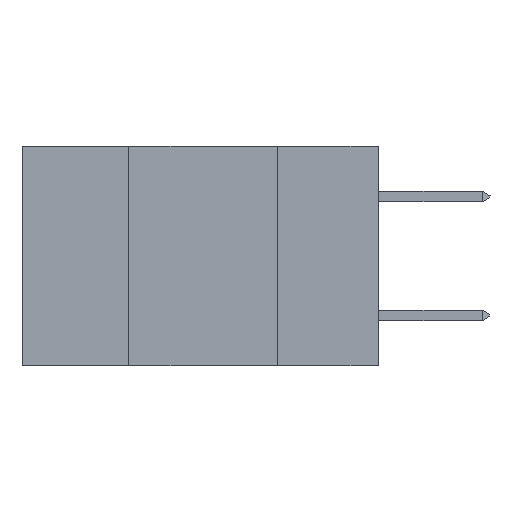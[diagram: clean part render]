
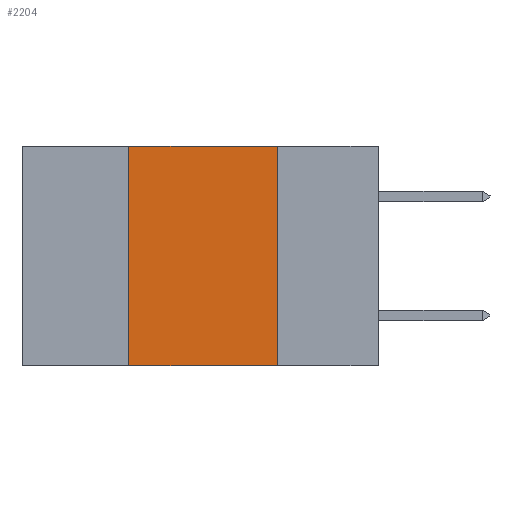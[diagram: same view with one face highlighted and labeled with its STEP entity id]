
A CAD part, left-side view. The second image highlights one B-rep face of the part: STEP entity #2204.
In plain terms, the highlighted planar face has unit normal (-1, 0, 0).
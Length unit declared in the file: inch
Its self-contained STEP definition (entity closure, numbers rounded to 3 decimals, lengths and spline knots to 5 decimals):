
#154 = ORIENTED_EDGE ( 'NONE', *, *, #9195, .F. ) ;
#379 = DIRECTION ( 'NONE',  ( 0., 0., 1. ) ) ;
#557 = EDGE_CURVE ( 'NONE', #3287, #9717, #8449, .T. ) ;
#773 = VECTOR ( 'NONE', #4101, 39.37008 ) ;
#999 = LINE ( 'NONE', #1804, #9194 ) ;
#1150 = DIRECTION ( 'NONE',  ( 0., 0., -1. ) ) ;
#1745 = DIRECTION ( 'NONE',  ( 0., -1., 0. ) ) ;
#1804 = CARTESIAN_POINT ( 'NONE',  ( 0., 0.6, -0.37 ) ) ;
#1882 = EDGE_LOOP ( 'NONE', ( #5538, #154, #5815, #4327 ) ) ;
#2204 = ADVANCED_FACE ( 'NONE', ( #4510 ), #5127, .F. ) ;
#2981 = VECTOR ( 'NONE', #5405, 39.37008 ) ;
#3287 = VERTEX_POINT ( 'NONE', #4253 ) ;
#4101 = DIRECTION ( 'NONE',  ( 0., -1., 0. ) ) ;
#4253 = CARTESIAN_POINT ( 'NONE',  ( 0., 0.42, -0.37 ) ) ;
#4327 = ORIENTED_EDGE ( 'NONE', *, *, #5433, .T. ) ;
#4399 = CARTESIAN_POINT ( 'NONE',  ( 0., 0.6, 0. ) ) ;
#4510 = FACE_OUTER_BOUND ( 'NONE', #1882, .T. ) ;
#4608 = VECTOR ( 'NONE', #379, 39.37008 ) ;
#4949 = VERTEX_POINT ( 'NONE', #4991 ) ;
#4969 = LINE ( 'NONE', #8846, #773 ) ;
#4991 = CARTESIAN_POINT ( 'NONE',  ( 0., 0.17, -0.37 ) ) ;
#5051 = AXIS2_PLACEMENT_3D ( 'NONE', #4399, #8329, #1150 ) ;
#5127 = PLANE ( 'NONE',  #5051 ) ;
#5405 = DIRECTION ( 'NONE',  ( 0., 0., -1. ) ) ;
#5433 = EDGE_CURVE ( 'NONE', #3287, #4949, #999, .T. ) ;
#5538 = ORIENTED_EDGE ( 'NONE', *, *, #9918, .F. ) ;
#5815 = ORIENTED_EDGE ( 'NONE', *, *, #557, .F. ) ;
#6698 = VERTEX_POINT ( 'NONE', #9164 ) ;
#8329 = DIRECTION ( 'NONE',  ( 1., 0., 0. ) ) ;
#8449 = LINE ( 'NONE', #10059, #4608 ) ;
#8752 = LINE ( 'NONE', #10229, #2981 ) ;
#8846 = CARTESIAN_POINT ( 'NONE',  ( 0., 0.6, 0. ) ) ;
#9127 = CARTESIAN_POINT ( 'NONE',  ( 0., 0.42, 0. ) ) ;
#9164 = CARTESIAN_POINT ( 'NONE',  ( 0., 0.17, 0. ) ) ;
#9194 = VECTOR ( 'NONE', #1745, 39.37008 ) ;
#9195 = EDGE_CURVE ( 'NONE', #9717, #6698, #4969, .T. ) ;
#9717 = VERTEX_POINT ( 'NONE', #9127 ) ;
#9918 = EDGE_CURVE ( 'NONE', #6698, #4949, #8752, .T. ) ;
#10059 = CARTESIAN_POINT ( 'NONE',  ( 0., 0.42, -0.37 ) ) ;
#10229 = CARTESIAN_POINT ( 'NONE',  ( 0., 0.17, -0.37 ) ) ;
